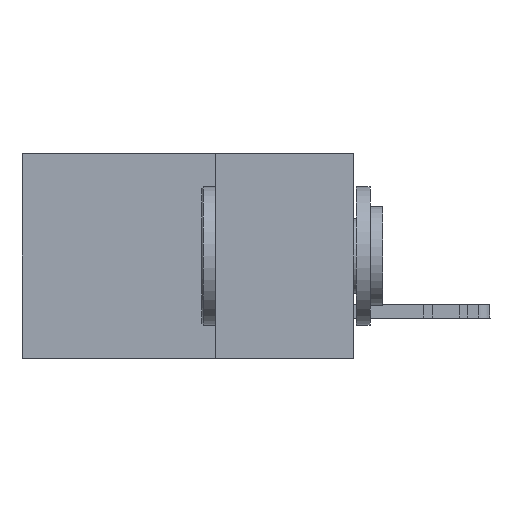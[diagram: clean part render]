
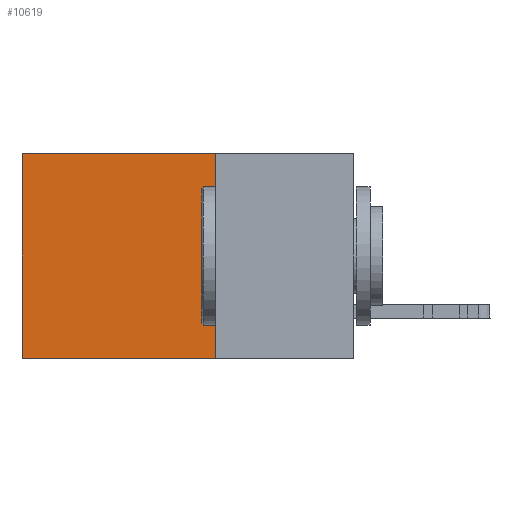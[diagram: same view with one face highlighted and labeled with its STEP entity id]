
A CAD part, left-side view. The second image highlights one B-rep face of the part: STEP entity #10619.
In plain terms, the highlighted planar face has unit normal (-1, 0, 0).
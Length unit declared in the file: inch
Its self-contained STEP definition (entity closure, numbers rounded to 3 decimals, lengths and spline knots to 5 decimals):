
#2110 = VERTEX_POINT ( 'NONE', #29767 ) ;
#2381 = EDGE_LOOP ( 'NONE', ( #11395, #36109, #34304, #6400 ) ) ;
#4132 = AXIS2_PLACEMENT_3D ( 'NONE', #37897, #45005, #20975 ) ;
#6189 = CARTESIAN_POINT ( 'NONE',  ( 0.2875, 0.6, 0. ) ) ;
#6400 = ORIENTED_EDGE ( 'NONE', *, *, #28471, .T. ) ;
#7531 = EDGE_CURVE ( 'NONE', #43948, #2110, #11765, .T. ) ;
#8957 = VECTOR ( 'NONE', #39640, 39.37008 ) ;
#10017 = FACE_OUTER_BOUND ( 'NONE', #2381, .T. ) ;
#10619 = ADVANCED_FACE ( 'NONE', ( #10017 ), #17553, .F. ) ;
#11395 = ORIENTED_EDGE ( 'NONE', *, *, #32453, .T. ) ;
#11765 = LINE ( 'NONE', #25682, #8957 ) ;
#12361 = VECTOR ( 'NONE', #14654, 39.37008 ) ;
#14597 = EDGE_CURVE ( 'NONE', #32630, #43948, #26775, .T. ) ;
#14654 = DIRECTION ( 'NONE',  ( 0., 1., 0. ) ) ;
#17553 = PLANE ( 'NONE',  #4132 ) ;
#17599 = CARTESIAN_POINT ( 'NONE',  ( 0.2875, 0.25, -0.37 ) ) ;
#20975 = DIRECTION ( 'NONE',  ( 0., 0., -1. ) ) ;
#25371 = LINE ( 'NONE', #36362, #12361 ) ;
#25428 = VECTOR ( 'NONE', #37304, 39.37008 ) ;
#25682 = CARTESIAN_POINT ( 'NONE',  ( 0.2875, 0.25, -0.37 ) ) ;
#26775 = LINE ( 'NONE', #40958, #25428 ) ;
#28471 = EDGE_CURVE ( 'NONE', #32630, #28564, #25371, .T. ) ;
#28564 = VERTEX_POINT ( 'NONE', #6189 ) ;
#29767 = CARTESIAN_POINT ( 'NONE',  ( 0.2875, 0.6, -0.37 ) ) ;
#32212 = VECTOR ( 'NONE', #33009, 39.37008 ) ;
#32453 = EDGE_CURVE ( 'NONE', #28564, #2110, #43752, .T. ) ;
#32630 = VERTEX_POINT ( 'NONE', #45112 ) ;
#33009 = DIRECTION ( 'NONE',  ( 0., 0., -1. ) ) ;
#34304 = ORIENTED_EDGE ( 'NONE', *, *, #14597, .F. ) ;
#36109 = ORIENTED_EDGE ( 'NONE', *, *, #7531, .F. ) ;
#36362 = CARTESIAN_POINT ( 'NONE',  ( 0.2875, 0.25, 0. ) ) ;
#36892 = CARTESIAN_POINT ( 'NONE',  ( 0.2875, 0.6, 0. ) ) ;
#37304 = DIRECTION ( 'NONE',  ( 0., 0., -1. ) ) ;
#37897 = CARTESIAN_POINT ( 'NONE',  ( 0.2875, 0.25, 0. ) ) ;
#39640 = DIRECTION ( 'NONE',  ( 0., 1., 0. ) ) ;
#40958 = CARTESIAN_POINT ( 'NONE',  ( 0.2875, 0.25, 0. ) ) ;
#43752 = LINE ( 'NONE', #36892, #32212 ) ;
#43948 = VERTEX_POINT ( 'NONE', #17599 ) ;
#45005 = DIRECTION ( 'NONE',  ( 1., 0., 0. ) ) ;
#45112 = CARTESIAN_POINT ( 'NONE',  ( 0.2875, 0.25, 0. ) ) ;
